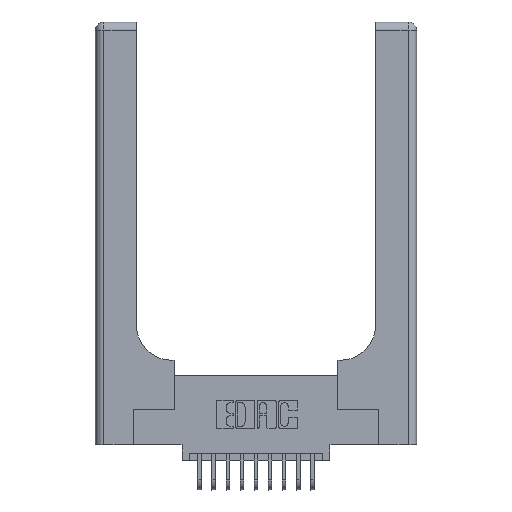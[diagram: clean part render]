
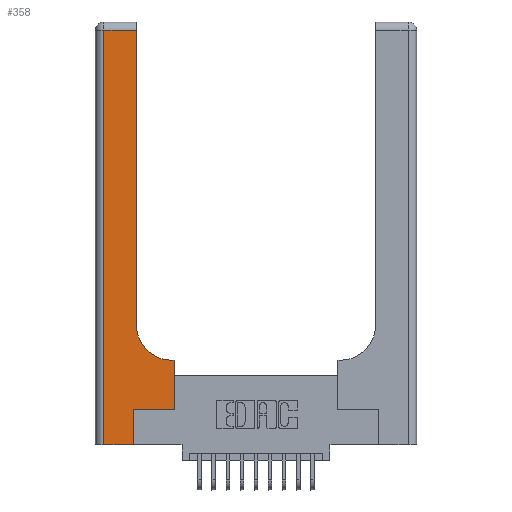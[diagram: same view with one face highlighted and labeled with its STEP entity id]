
A CAD part, top view. The second image highlights one B-rep face of the part: STEP entity #358.
In plain terms, the highlighted planar face has unit normal (0, 0, 1).
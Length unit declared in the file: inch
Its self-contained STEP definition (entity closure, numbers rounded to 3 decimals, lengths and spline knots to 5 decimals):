
#350 = CARTESIAN_POINT ( 'NONE',  ( 0., 2.94, 0.37 ) ) ;
#358 = ADVANCED_FACE ( 'NONE', ( #5659 ), #10910, .F. ) ;
#652 = ORIENTED_EDGE ( 'NONE', *, *, #3886, .T. ) ;
#710 = VERTEX_POINT ( 'NONE', #5119 ) ;
#849 = VERTEX_POINT ( 'NONE', #13493 ) ;
#1447 = VECTOR ( 'NONE', #16345, 39.37008 ) ;
#1510 = LINE ( 'NONE', #4525, #2653 ) ;
#1666 = DIRECTION ( 'NONE',  ( -1., 0., 0. ) ) ;
#2223 = EDGE_LOOP ( 'NONE', ( #10775, #3383, #9108, #11978, #14918, #652, #11428, #10343, #12846 ) ) ;
#2653 = VECTOR ( 'NONE', #15796, 39.37008 ) ;
#2846 = EDGE_CURVE ( 'NONE', #849, #4801, #6883, .T. ) ;
#3007 = DIRECTION ( 'NONE',  ( 0., 1., 0. ) ) ;
#3059 = DIRECTION ( 'NONE',  ( 0., 1., 0. ) ) ;
#3271 = CARTESIAN_POINT ( 'NONE',  ( 0.2915, 0.6, 0.37 ) ) ;
#3327 = DIRECTION ( 'NONE',  ( -1., 0., 0. ) ) ;
#3383 = ORIENTED_EDGE ( 'NONE', *, *, #2846, .T. ) ;
#3459 = VECTOR ( 'NONE', #3327, 39.37008 ) ;
#3886 = EDGE_CURVE ( 'NONE', #9389, #7441, #9742, .T. ) ;
#4262 = CARTESIAN_POINT ( 'NONE',  ( 0.269, 0., 0.37 ) ) ;
#4525 = CARTESIAN_POINT ( 'NONE',  ( 0., 0., 0.37 ) ) ;
#4801 = VERTEX_POINT ( 'NONE', #16308 ) ;
#5119 = CARTESIAN_POINT ( 'NONE',  ( 0.2915, 0.85, 0.37 ) ) ;
#5211 = EDGE_CURVE ( 'NONE', #6942, #9389, #17929, .T. ) ;
#5216 = AXIS2_PLACEMENT_3D ( 'NONE', #16579, #12344, #8029 ) ;
#5659 = FACE_OUTER_BOUND ( 'NONE', #2223, .T. ) ;
#5875 = CARTESIAN_POINT ( 'NONE',  ( 0.5585, 0.25, 0.37 ) ) ;
#6043 = CARTESIAN_POINT ( 'NONE',  ( 0.06, 3., 0.37 ) ) ;
#6313 = CARTESIAN_POINT ( 'NONE',  ( 0.269, 0.25, 0.37 ) ) ;
#6360 = CARTESIAN_POINT ( 'NONE',  ( 0.269, 0., 0.37 ) ) ;
#6604 = AXIS2_PLACEMENT_3D ( 'NONE', #11528, #14617, #7345 ) ;
#6663 = VECTOR ( 'NONE', #1666, 39.37008 ) ;
#6883 = LINE ( 'NONE', #350, #6663 ) ;
#6942 = VERTEX_POINT ( 'NONE', #6360 ) ;
#6972 = DIRECTION ( 'NONE',  ( 0., 1., 0. ) ) ;
#7345 = DIRECTION ( 'NONE',  ( 1., 0., 0. ) ) ;
#7441 = VERTEX_POINT ( 'NONE', #16368 ) ;
#7761 = CARTESIAN_POINT ( 'NONE',  ( 0.269, 0.25, 0.37 ) ) ;
#8029 = DIRECTION ( 'NONE',  ( -1., 0., 0. ) ) ;
#8821 = LINE ( 'NONE', #14053, #12172 ) ;
#8915 = DIRECTION ( 'NONE',  ( 0., -1., 0. ) ) ;
#8939 = VERTEX_POINT ( 'NONE', #15136 ) ;
#9036 = EDGE_CURVE ( 'NONE', #8939, #6942, #1510, .T. ) ;
#9108 = ORIENTED_EDGE ( 'NONE', *, *, #15133, .T. ) ;
#9228 = CARTESIAN_POINT ( 'NONE',  ( 0.5415, 0.6, 0.37 ) ) ;
#9389 = VERTEX_POINT ( 'NONE', #7761 ) ;
#9713 = EDGE_CURVE ( 'NONE', #7441, #12230, #18032, .T. ) ;
#9742 = LINE ( 'NONE', #6313, #1447 ) ;
#10050 = LINE ( 'NONE', #6043, #16525 ) ;
#10185 = CIRCLE ( 'NONE', #6604, 0.25 ) ;
#10343 = ORIENTED_EDGE ( 'NONE', *, *, #12237, .T. ) ;
#10451 = VECTOR ( 'NONE', #3059, 39.37008 ) ;
#10775 = ORIENTED_EDGE ( 'NONE', *, *, #12513, .T. ) ;
#10910 = PLANE ( 'NONE',  #5216 ) ;
#11428 = ORIENTED_EDGE ( 'NONE', *, *, #9713, .T. ) ;
#11528 = CARTESIAN_POINT ( 'NONE',  ( 0.5415, 0.85, 0.37 ) ) ;
#11716 = VERTEX_POINT ( 'NONE', #9228 ) ;
#11978 = ORIENTED_EDGE ( 'NONE', *, *, #9036, .T. ) ;
#12172 = VECTOR ( 'NONE', #6972, 39.37008 ) ;
#12230 = VERTEX_POINT ( 'NONE', #13309 ) ;
#12237 = EDGE_CURVE ( 'NONE', #12230, #11716, #12812, .T. ) ;
#12344 = DIRECTION ( 'NONE',  ( 0., 0., -1. ) ) ;
#12513 = EDGE_CURVE ( 'NONE', #710, #849, #8821, .T. ) ;
#12812 = LINE ( 'NONE', #3271, #3459 ) ;
#12846 = ORIENTED_EDGE ( 'NONE', *, *, #18472, .T. ) ;
#13309 = CARTESIAN_POINT ( 'NONE',  ( 0.5585, 0.6, 0.37 ) ) ;
#13493 = CARTESIAN_POINT ( 'NONE',  ( 0.2915, 2.94, 0.37 ) ) ;
#14053 = CARTESIAN_POINT ( 'NONE',  ( 0.2915, 3., 0.37 ) ) ;
#14138 = VECTOR ( 'NONE', #3007, 39.37008 ) ;
#14617 = DIRECTION ( 'NONE',  ( 0., 0., -1. ) ) ;
#14918 = ORIENTED_EDGE ( 'NONE', *, *, #5211, .T. ) ;
#15133 = EDGE_CURVE ( 'NONE', #4801, #8939, #10050, .T. ) ;
#15136 = CARTESIAN_POINT ( 'NONE',  ( 0.06, 0., 0.37 ) ) ;
#15796 = DIRECTION ( 'NONE',  ( 1., 0., 0. ) ) ;
#16308 = CARTESIAN_POINT ( 'NONE',  ( 0.06, 2.94, 0.37 ) ) ;
#16345 = DIRECTION ( 'NONE',  ( 1., 0., 0. ) ) ;
#16368 = CARTESIAN_POINT ( 'NONE',  ( 0.5585, 0.25, 0.37 ) ) ;
#16525 = VECTOR ( 'NONE', #8915, 39.37008 ) ;
#16579 = CARTESIAN_POINT ( 'NONE',  ( 0., 3., 0.37 ) ) ;
#17929 = LINE ( 'NONE', #4262, #14138 ) ;
#18032 = LINE ( 'NONE', #5875, #10451 ) ;
#18472 = EDGE_CURVE ( 'NONE', #11716, #710, #10185, .T. ) ;
